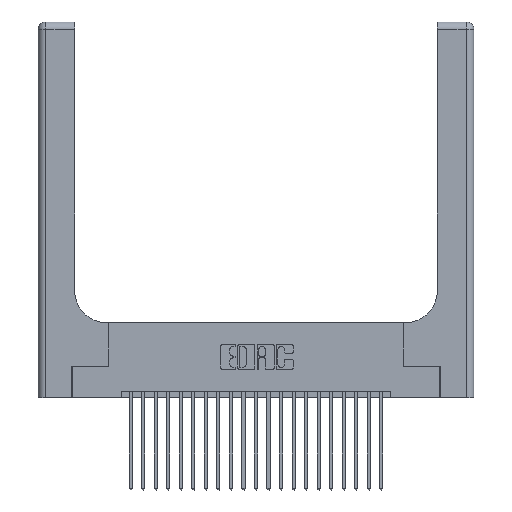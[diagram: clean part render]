
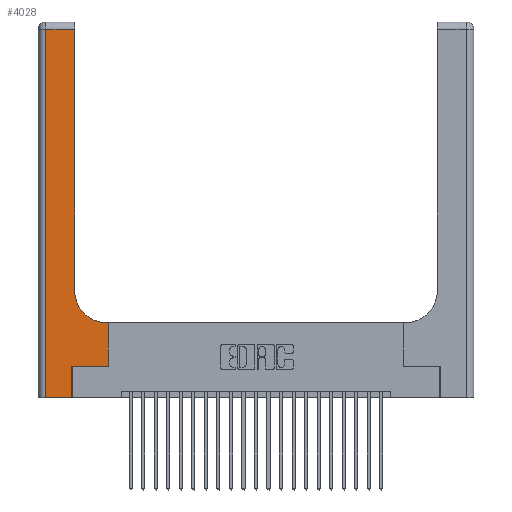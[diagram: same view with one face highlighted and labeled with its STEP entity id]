
A CAD part, top view. The second image highlights one B-rep face of the part: STEP entity #4028.
In plain terms, the highlighted planar face has unit normal (0, 0, 1).
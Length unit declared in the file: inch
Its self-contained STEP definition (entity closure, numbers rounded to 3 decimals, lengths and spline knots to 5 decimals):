
#558 = LINE ( 'NONE', #10521, #10066 ) ;
#1184 = VERTEX_POINT ( 'NONE', #8252 ) ;
#1259 = CARTESIAN_POINT ( 'NONE',  ( 0.5585, 0.25, 0.37 ) ) ;
#1356 = VERTEX_POINT ( 'NONE', #3203 ) ;
#1373 = EDGE_CURVE ( 'NONE', #1356, #3557, #17586, .T. ) ;
#1891 = VECTOR ( 'NONE', #21364, 39.37008 ) ;
#1943 = VERTEX_POINT ( 'NONE', #14810 ) ;
#2501 = LINE ( 'NONE', #19451, #1891 ) ;
#3061 = CARTESIAN_POINT ( 'NONE',  ( 0.06, 2.94, 0.37 ) ) ;
#3149 = EDGE_CURVE ( 'NONE', #24096, #16700, #6575, .T. ) ;
#3203 = CARTESIAN_POINT ( 'NONE',  ( 0.5415, 0.6, 0.37 ) ) ;
#3215 = EDGE_CURVE ( 'NONE', #1184, #13892, #24261, .T. ) ;
#3224 = FACE_OUTER_BOUND ( 'NONE', #21111, .T. ) ;
#3246 = LINE ( 'NONE', #10256, #23332 ) ;
#3516 = EDGE_CURVE ( 'NONE', #1943, #1184, #3246, .T. ) ;
#3557 = VERTEX_POINT ( 'NONE', #14124 ) ;
#4028 = ADVANCED_FACE ( 'NONE', ( #3224 ), #18117, .F. ) ;
#4345 = ORIENTED_EDGE ( 'NONE', *, *, #8547, .T. ) ;
#4396 = CARTESIAN_POINT ( 'NONE',  ( 0.5585, 0.25, 0.37 ) ) ;
#4467 = ORIENTED_EDGE ( 'NONE', *, *, #15261, .T. ) ;
#4716 = LINE ( 'NONE', #4396, #24168 ) ;
#4816 = VECTOR ( 'NONE', #9164, 39.37008 ) ;
#4905 = CARTESIAN_POINT ( 'NONE',  ( 0., 3., 0.37 ) ) ;
#4953 = EDGE_CURVE ( 'NONE', #13892, #15420, #22691, .T. ) ;
#5382 = CARTESIAN_POINT ( 'NONE',  ( 0.269, 0., 0.37 ) ) ;
#5514 = CARTESIAN_POINT ( 'NONE',  ( 0.2915, 2.94, 0.37 ) ) ;
#5728 = VECTOR ( 'NONE', #15270, 39.37008 ) ;
#6206 = DIRECTION ( 'NONE',  ( 0., 1., 0. ) ) ;
#6575 = LINE ( 'NONE', #10806, #16022 ) ;
#7091 = CARTESIAN_POINT ( 'NONE',  ( 0.5415, 0.85, 0.37 ) ) ;
#8252 = CARTESIAN_POINT ( 'NONE',  ( 0.269, 0., 0.37 ) ) ;
#8547 = EDGE_CURVE ( 'NONE', #16700, #1943, #20785, .T. ) ;
#8997 = DIRECTION ( 'NONE',  ( 1., 0., 0. ) ) ;
#9164 = DIRECTION ( 'NONE',  ( 0., 1., 0. ) ) ;
#10066 = VECTOR ( 'NONE', #12393, 39.37008 ) ;
#10256 = CARTESIAN_POINT ( 'NONE',  ( 0., 0., 0.37 ) ) ;
#10521 = CARTESIAN_POINT ( 'NONE',  ( 0.2915, 0.6, 0.37 ) ) ;
#10570 = DIRECTION ( 'NONE',  ( 0., 0., -1. ) ) ;
#10806 = CARTESIAN_POINT ( 'NONE',  ( 0., 2.94, 0.37 ) ) ;
#11202 = ORIENTED_EDGE ( 'NONE', *, *, #3149, .T. ) ;
#12393 = DIRECTION ( 'NONE',  ( -1., 0., 0. ) ) ;
#12671 = DIRECTION ( 'NONE',  ( -1., 0., 0. ) ) ;
#13704 = EDGE_CURVE ( 'NONE', #23577, #1356, #558, .T. ) ;
#13892 = VERTEX_POINT ( 'NONE', #20787 ) ;
#14124 = CARTESIAN_POINT ( 'NONE',  ( 0.2915, 0.85, 0.37 ) ) ;
#14810 = CARTESIAN_POINT ( 'NONE',  ( 0.06, 0., 0.37 ) ) ;
#14899 = ORIENTED_EDGE ( 'NONE', *, *, #3215, .T. ) ;
#14907 = CARTESIAN_POINT ( 'NONE',  ( 0.269, 0.25, 0.37 ) ) ;
#15261 = EDGE_CURVE ( 'NONE', #15420, #23577, #4716, .T. ) ;
#15270 = DIRECTION ( 'NONE',  ( 0., -1., 0. ) ) ;
#15323 = AXIS2_PLACEMENT_3D ( 'NONE', #4905, #10570, #23772 ) ;
#15420 = VERTEX_POINT ( 'NONE', #1259 ) ;
#16022 = VECTOR ( 'NONE', #12671, 39.37008 ) ;
#16100 = ORIENTED_EDGE ( 'NONE', *, *, #3516, .T. ) ;
#16700 = VERTEX_POINT ( 'NONE', #3061 ) ;
#17101 = CARTESIAN_POINT ( 'NONE',  ( 0.06, 3., 0.37 ) ) ;
#17586 = CIRCLE ( 'NONE', #24132, 0.25 ) ;
#18117 = PLANE ( 'NONE',  #15323 ) ;
#18978 = CARTESIAN_POINT ( 'NONE',  ( 0.5585, 0.6, 0.37 ) ) ;
#19202 = ORIENTED_EDGE ( 'NONE', *, *, #4953, .T. ) ;
#19451 = CARTESIAN_POINT ( 'NONE',  ( 0.2915, 3., 0.37 ) ) ;
#20179 = ORIENTED_EDGE ( 'NONE', *, *, #22587, .T. ) ;
#20319 = DIRECTION ( 'NONE',  ( 0., 0., -1. ) ) ;
#20785 = LINE ( 'NONE', #17101, #5728 ) ;
#20787 = CARTESIAN_POINT ( 'NONE',  ( 0.269, 0.25, 0.37 ) ) ;
#21111 = EDGE_LOOP ( 'NONE', ( #20179, #11202, #4345, #16100, #14899, #19202, #4467, #23668, #22233 ) ) ;
#21364 = DIRECTION ( 'NONE',  ( 0., 1., 0. ) ) ;
#22119 = VECTOR ( 'NONE', #24371, 39.37008 ) ;
#22233 = ORIENTED_EDGE ( 'NONE', *, *, #1373, .T. ) ;
#22587 = EDGE_CURVE ( 'NONE', #3557, #24096, #2501, .T. ) ;
#22691 = LINE ( 'NONE', #14907, #22119 ) ;
#23332 = VECTOR ( 'NONE', #23470, 39.37008 ) ;
#23470 = DIRECTION ( 'NONE',  ( 1., 0., 0. ) ) ;
#23577 = VERTEX_POINT ( 'NONE', #18978 ) ;
#23668 = ORIENTED_EDGE ( 'NONE', *, *, #13704, .T. ) ;
#23772 = DIRECTION ( 'NONE',  ( -1., 0., 0. ) ) ;
#24096 = VERTEX_POINT ( 'NONE', #5514 ) ;
#24132 = AXIS2_PLACEMENT_3D ( 'NONE', #7091, #20319, #8997 ) ;
#24168 = VECTOR ( 'NONE', #6206, 39.37008 ) ;
#24261 = LINE ( 'NONE', #5382, #4816 ) ;
#24371 = DIRECTION ( 'NONE',  ( 1., 0., 0. ) ) ;
